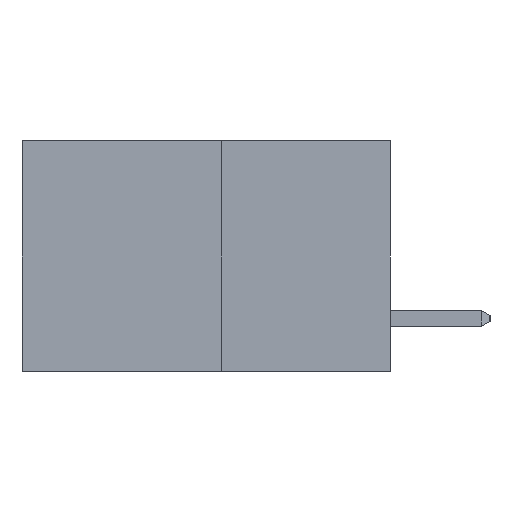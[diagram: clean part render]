
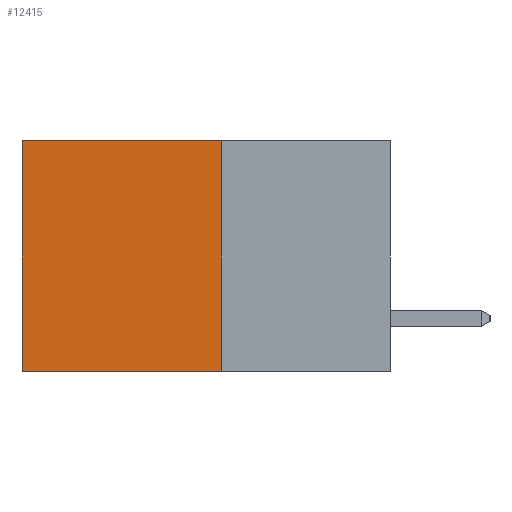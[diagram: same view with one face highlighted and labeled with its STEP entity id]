
A CAD part, left-side view. The second image highlights one B-rep face of the part: STEP entity #12415.
In plain terms, the highlighted planar face has unit normal (-1, 0, 0).
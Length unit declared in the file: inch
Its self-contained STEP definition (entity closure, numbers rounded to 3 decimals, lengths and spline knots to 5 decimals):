
#133 = LINE ( 'NONE', #1272, #10275 ) ;
#274 = CARTESIAN_POINT ( 'NONE',  ( 0.277, 0.27, 0. ) ) ;
#346 = EDGE_LOOP ( 'NONE', ( #1351, #11453, #11418, #1118 ) ) ;
#1118 = ORIENTED_EDGE ( 'NONE', *, *, #10339, .T. ) ;
#1272 = CARTESIAN_POINT ( 'NONE',  ( 0.277, 0.59, -0.37 ) ) ;
#1278 = VECTOR ( 'NONE', #8551, 39.37008 ) ;
#1351 = ORIENTED_EDGE ( 'NONE', *, *, #5099, .T. ) ;
#1854 = CARTESIAN_POINT ( 'NONE',  ( 0.277, 0.27, 0. ) ) ;
#1998 = CARTESIAN_POINT ( 'NONE',  ( 0.277, 0.59, -0.37 ) ) ;
#2451 = DIRECTION ( 'NONE',  ( 0., 0., -1. ) ) ;
#2881 = LINE ( 'NONE', #11793, #6917 ) ;
#3422 = VERTEX_POINT ( 'NONE', #11398 ) ;
#3529 = DIRECTION ( 'NONE',  ( 1., 0., 0. ) ) ;
#4531 = VECTOR ( 'NONE', #9713, 39.37008 ) ;
#4611 = CARTESIAN_POINT ( 'NONE',  ( 0.277, 0.27, -0.37 ) ) ;
#5099 = EDGE_CURVE ( 'NONE', #3422, #6046, #133, .T. ) ;
#5487 = PLANE ( 'NONE',  #7301 ) ;
#5565 = CARTESIAN_POINT ( 'NONE',  ( 0.277, 0.27, -0.37 ) ) ;
#5654 = DIRECTION ( 'NONE',  ( 0., 0., -1. ) ) ;
#6046 = VERTEX_POINT ( 'NONE', #1998 ) ;
#6917 = VECTOR ( 'NONE', #2451, 39.37008 ) ;
#7301 = AXIS2_PLACEMENT_3D ( 'NONE', #9412, #3529, #10346 ) ;
#7658 = EDGE_CURVE ( 'NONE', #12230, #10782, #2881, .T. ) ;
#8551 = DIRECTION ( 'NONE',  ( 0., 1., 0. ) ) ;
#8830 = LINE ( 'NONE', #4611, #1278 ) ;
#9412 = CARTESIAN_POINT ( 'NONE',  ( 0.277, 0.27, -0.37 ) ) ;
#9713 = DIRECTION ( 'NONE',  ( 0., 1., 0. ) ) ;
#10275 = VECTOR ( 'NONE', #5654, 39.37008 ) ;
#10339 = EDGE_CURVE ( 'NONE', #12230, #3422, #11891, .T. ) ;
#10346 = DIRECTION ( 'NONE',  ( 0., 0., -1. ) ) ;
#10782 = VERTEX_POINT ( 'NONE', #5565 ) ;
#10799 = EDGE_CURVE ( 'NONE', #10782, #6046, #8830, .T. ) ;
#11098 = FACE_OUTER_BOUND ( 'NONE', #346, .T. ) ;
#11398 = CARTESIAN_POINT ( 'NONE',  ( 0.277, 0.59, 0. ) ) ;
#11418 = ORIENTED_EDGE ( 'NONE', *, *, #7658, .F. ) ;
#11453 = ORIENTED_EDGE ( 'NONE', *, *, #10799, .F. ) ;
#11793 = CARTESIAN_POINT ( 'NONE',  ( 0.277, 0.27, -0.37 ) ) ;
#11891 = LINE ( 'NONE', #1854, #4531 ) ;
#12230 = VERTEX_POINT ( 'NONE', #274 ) ;
#12415 = ADVANCED_FACE ( 'NONE', ( #11098 ), #5487, .F. ) ;
